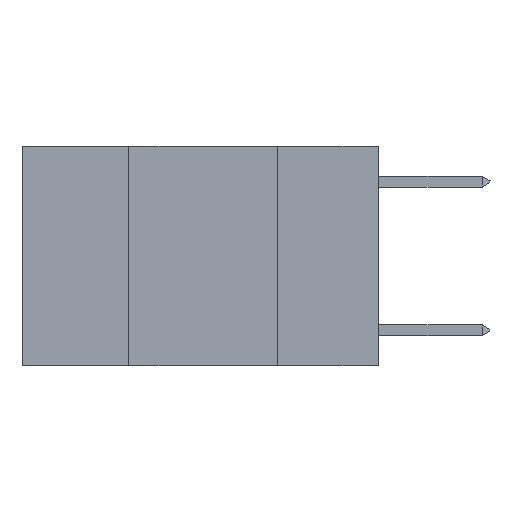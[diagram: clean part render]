
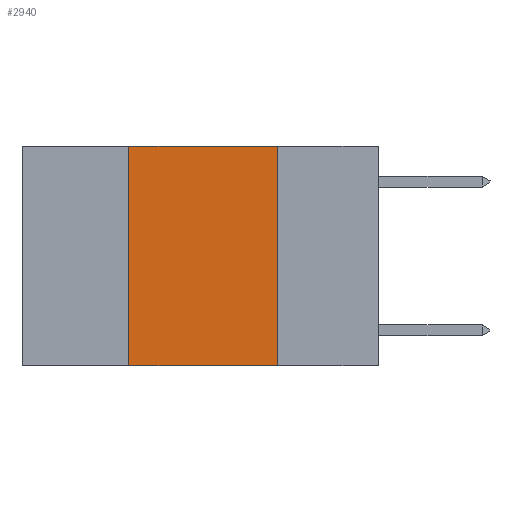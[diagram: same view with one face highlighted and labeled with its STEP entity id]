
A CAD part, left-side view. The second image highlights one B-rep face of the part: STEP entity #2940.
In plain terms, the highlighted planar face has unit normal (-1, 0, 0).
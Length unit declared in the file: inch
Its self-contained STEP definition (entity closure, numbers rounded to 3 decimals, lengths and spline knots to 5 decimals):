
#39 = CARTESIAN_POINT ( 'NONE',  ( 0., 0.42, 0. ) ) ;
#984 = DIRECTION ( 'NONE',  ( 1., 0., 0. ) ) ;
#1303 = VECTOR ( 'NONE', #6512, 39.37008 ) ;
#2423 = VERTEX_POINT ( 'NONE', #2999 ) ;
#2471 = DIRECTION ( 'NONE',  ( 0., 0., -1. ) ) ;
#2598 = VECTOR ( 'NONE', #3303, 39.37008 ) ;
#2661 = LINE ( 'NONE', #4480, #6582 ) ;
#2899 = CARTESIAN_POINT ( 'NONE',  ( 0., 0.42, -0.37 ) ) ;
#2940 = ADVANCED_FACE ( 'NONE', ( #5138 ), #9859, .F. ) ;
#2999 = CARTESIAN_POINT ( 'NONE',  ( 0., 0.17, 0. ) ) ;
#3303 = DIRECTION ( 'NONE',  ( 0., -1., 0. ) ) ;
#3669 = VERTEX_POINT ( 'NONE', #4677 ) ;
#4033 = VERTEX_POINT ( 'NONE', #39 ) ;
#4480 = CARTESIAN_POINT ( 'NONE',  ( 0., 0.6, 0. ) ) ;
#4653 = LINE ( 'NONE', #7270, #2598 ) ;
#4677 = CARTESIAN_POINT ( 'NONE',  ( 0., 0.17, -0.37 ) ) ;
#4719 = EDGE_CURVE ( 'NONE', #7010, #4033, #6000, .T. ) ;
#4921 = AXIS2_PLACEMENT_3D ( 'NONE', #4926, #984, #6536 ) ;
#4926 = CARTESIAN_POINT ( 'NONE',  ( 0., 0.6, 0. ) ) ;
#5138 = FACE_OUTER_BOUND ( 'NONE', #6771, .T. ) ;
#5539 = ORIENTED_EDGE ( 'NONE', *, *, #6636, .F. ) ;
#5695 = CARTESIAN_POINT ( 'NONE',  ( 0., 0.42, 0. ) ) ;
#6000 = LINE ( 'NONE', #5695, #1303 ) ;
#6046 = DIRECTION ( 'NONE',  ( 0., -1., 0. ) ) ;
#6512 = DIRECTION ( 'NONE',  ( 0., 0., 1. ) ) ;
#6536 = DIRECTION ( 'NONE',  ( 0., 0., -1. ) ) ;
#6582 = VECTOR ( 'NONE', #6046, 39.37008 ) ;
#6636 = EDGE_CURVE ( 'NONE', #4033, #2423, #2661, .T. ) ;
#6771 = EDGE_LOOP ( 'NONE', ( #9701, #5539, #7716, #9940 ) ) ;
#6800 = EDGE_CURVE ( 'NONE', #2423, #3669, #10309, .T. ) ;
#7010 = VERTEX_POINT ( 'NONE', #2899 ) ;
#7211 = CARTESIAN_POINT ( 'NONE',  ( 0., 0.17, 0. ) ) ;
#7270 = CARTESIAN_POINT ( 'NONE',  ( 0., 0.6, -0.37 ) ) ;
#7716 = ORIENTED_EDGE ( 'NONE', *, *, #4719, .F. ) ;
#8343 = EDGE_CURVE ( 'NONE', #7010, #3669, #4653, .T. ) ;
#9701 = ORIENTED_EDGE ( 'NONE', *, *, #6800, .F. ) ;
#9859 = PLANE ( 'NONE',  #4921 ) ;
#9940 = ORIENTED_EDGE ( 'NONE', *, *, #8343, .T. ) ;
#10309 = LINE ( 'NONE', #7211, #10543 ) ;
#10543 = VECTOR ( 'NONE', #2471, 39.37008 ) ;
